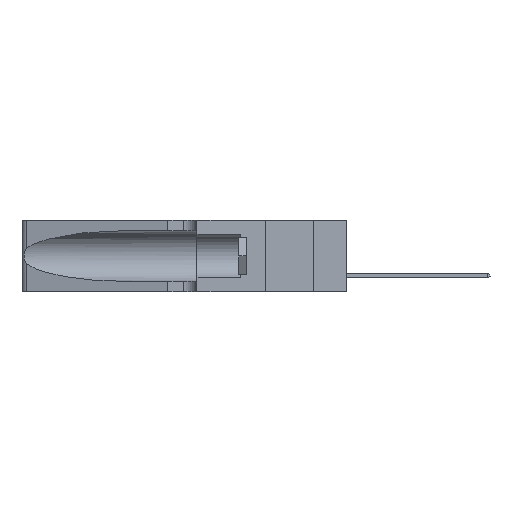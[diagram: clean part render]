
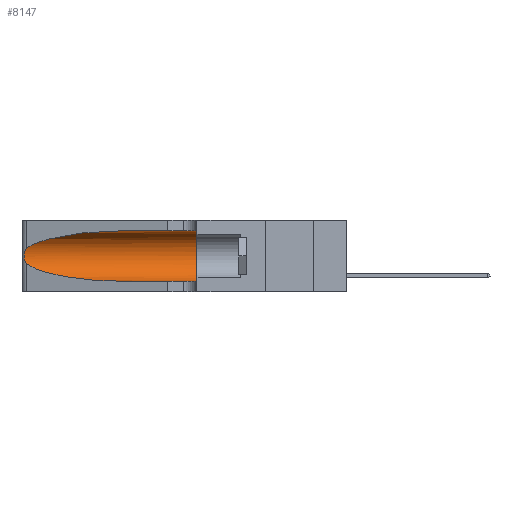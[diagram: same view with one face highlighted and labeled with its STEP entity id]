
A CAD part, left-side view. The second image highlights one B-rep face of the part: STEP entity #8147.
In plain terms, the highlighted cylindrical face has radius 3.308 mm (diameter 6.617 mm), a partial arc.
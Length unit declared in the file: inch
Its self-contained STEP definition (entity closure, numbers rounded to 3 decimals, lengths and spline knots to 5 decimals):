
#199 = FACE_OUTER_BOUND ( 'NONE', #6967, .T. ) ;
#1087 = CARTESIAN_POINT ( 'NONE',  ( 0.25487, 1.22718, 0.14631 ) ) ;
#1635 = CARTESIAN_POINT ( 'NONE',  ( 0.26018, 1.23835, 0.19895 ) ) ;
#2266 = ORIENTED_EDGE ( 'NONE', *, *, #4093, .T. ) ;
#2772 = CARTESIAN_POINT ( 'NONE',  ( 0.18966, 0.96281, 0.31525 ) ) ;
#2978 = CARTESIAN_POINT ( 'NONE',  ( 0.1305, 1.61858, 0.185 ) ) ;
#3443 = DIRECTION ( 'NONE',  ( 0., 1., 0. ) ) ;
#4093 = EDGE_CURVE ( 'NONE', #20057, #7512, #4691, .T. ) ;
#4691 = B_SPLINE_CURVE_WITH_KNOTS ( 'NONE', 3,
 ( #38558, #27583, #8957, #8781, #42356, #1635, #16392, #19839, #23615, #35313, #12773, #34964, #24465, #20704 ),
 .UNSPECIFIED., .F., .F.,
 ( 4, 2, 2, 2, 2, 2, 4 ),
 ( 0., 0.00027, 0.00053, 0.00107, 0.0016, 0.00187, 0.00214 ),
 .UNSPECIFIED. ) ;
#6109 = CARTESIAN_POINT ( 'NONE',  ( 0.25487, 1.22718, 0.22369 ) ) ;
#6454 = EDGE_CURVE ( 'NONE', #41723, #23977, #20462, .T. ) ;
#6967 = EDGE_LOOP ( 'NONE', ( #35686, #2266, #26978, #8843, #28911, #47625 ) ) ;
#7424 = CARTESIAN_POINT ( 'NONE',  ( 0.25487, 1.22718, 0.14631 ) ) ;
#7512 = VERTEX_POINT ( 'NONE', #7424 ) ;
#8147 = ADVANCED_FACE ( 'NONE', ( #199 ), #42537, .F. ) ;
#8781 = CARTESIAN_POINT ( 'NONE',  ( 0.25787, 1.23484, 0.2124 ) ) ;
#8843 = ORIENTED_EDGE ( 'NONE', *, *, #16078, .T. ) ;
#8957 = CARTESIAN_POINT ( 'NONE',  ( 0.25639, 1.23184, 0.21858 ) ) ;
#10916 = CARTESIAN_POINT ( 'NONE',  ( 0.1305, 0.35, 0.31525 ) ) ;
#12492 = DIRECTION ( 'NONE',  ( 0., -1., 0. ) ) ;
#12773 = CARTESIAN_POINT ( 'NONE',  ( 0.25789, 1.23486, 0.15765 ) ) ;
#12911 = LINE ( 'NONE', #35363, #38768 ) ;
#14139 = DIRECTION ( 'NONE',  ( 0., -1., 0. ) ) ;
#14301 = CARTESIAN_POINT ( 'NONE',  ( 0.1305, 0.35, 0.185 ) ) ;
#15576 = EDGE_CURVE ( 'NONE', #7512, #38236, #43875, .T. ) ;
#16078 = EDGE_CURVE ( 'NONE', #38236, #23977, #12911, .T. ) ;
#16392 = CARTESIAN_POINT ( 'NONE',  ( 0.26075, 1.23896, 0.19203 ) ) ;
#16457 = AXIS2_PLACEMENT_3D ( 'NONE', #14301, #3443, #17728 ) ;
#17728 = DIRECTION ( 'NONE',  ( 0., 0., 1. ) ) ;
#18174 = CARTESIAN_POINT ( 'NONE',  ( 0.2373, 1.15595, 0.28018 ) ) ;
#18338 = CARTESIAN_POINT ( 'NONE',  ( 0.1305, 0.72297, 0.05475 ) ) ;
#19839 = CARTESIAN_POINT ( 'NONE',  ( 0.26075, 1.23896, 0.178 ) ) ;
#19980 = AXIS2_PLACEMENT_3D ( 'NONE', #2978, #14139, #43865 ) ;
#20057 = VERTEX_POINT ( 'NONE', #6109 ) ;
#20462 = CIRCLE ( 'NONE', #16457, 0.13025 ) ;
#20704 = CARTESIAN_POINT ( 'NONE',  ( 0.25487, 1.22718, 0.14631 ) ) ;
#21912 = EDGE_CURVE ( 'NONE', #36188, #41723, #32035, .T. ) ;
#23615 = CARTESIAN_POINT ( 'NONE',  ( 0.26017, 1.23833, 0.17102 ) ) ;
#23977 = VERTEX_POINT ( 'NONE', #47162 ) ;
#24465 = CARTESIAN_POINT ( 'NONE',  ( 0.25555, 1.22993, 0.14849 ) ) ;
#25260 = CARTESIAN_POINT ( 'NONE',  ( 0.1305, 0.72297, 0.31525 ) ) ;
#26978 = ORIENTED_EDGE ( 'NONE', *, *, #15576, .T. ) ;
#27405 = EDGE_CURVE ( 'NONE', #36188, #20057, #35108, .T. ) ;
#27583 = CARTESIAN_POINT ( 'NONE',  ( 0.25555, 1.22994, 0.2215 ) ) ;
#28911 = ORIENTED_EDGE ( 'NONE', *, *, #6454, .F. ) ;
#31157 = DIRECTION ( 'NONE',  ( 0., -1., 0. ) ) ;
#32035 = LINE ( 'NONE', #41721, #46117 ) ;
#34964 = CARTESIAN_POINT ( 'NONE',  ( 0.25639, 1.23186, 0.15144 ) ) ;
#35108 =( BOUNDED_CURVE ( )  B_SPLINE_CURVE ( 3, ( #25260, #2772, #18174, #40537 ),
 .UNSPECIFIED., .F., .F. ) 
 B_SPLINE_CURVE_WITH_KNOTS ( ( 4, 4 ),
 ( 1.5708, 2.84003 ),
 .UNSPECIFIED. ) 
 CURVE ( )  GEOMETRIC_REPRESENTATION_ITEM ( )  RATIONAL_B_SPLINE_CURVE ( ( 1., 0.87, 0.87, 1. ) ) 
 REPRESENTATION_ITEM ( '' )  );
#35313 = CARTESIAN_POINT ( 'NONE',  ( 0.25856, 1.23593, 0.16098 ) ) ;
#35363 = CARTESIAN_POINT ( 'NONE',  ( 0.1305, 1.61858, 0.05475 ) ) ;
#35686 = ORIENTED_EDGE ( 'NONE', *, *, #27405, .T. ) ;
#36188 = VERTEX_POINT ( 'NONE', #47766 ) ;
#38236 = VERTEX_POINT ( 'NONE', #18338 ) ;
#38558 = CARTESIAN_POINT ( 'NONE',  ( 0.25487, 1.22718, 0.22369 ) ) ;
#38768 = VECTOR ( 'NONE', #12492, 39.37008 ) ;
#38838 = CARTESIAN_POINT ( 'NONE',  ( 0.2373, 1.15595, 0.08982 ) ) ;
#40537 = CARTESIAN_POINT ( 'NONE',  ( 0.25487, 1.22718, 0.22369 ) ) ;
#41721 = CARTESIAN_POINT ( 'NONE',  ( 0.1305, 1.61858, 0.31525 ) ) ;
#41723 = VERTEX_POINT ( 'NONE', #10916 ) ;
#42013 = CARTESIAN_POINT ( 'NONE',  ( 0.1305, 0.72297, 0.05475 ) ) ;
#42356 = CARTESIAN_POINT ( 'NONE',  ( 0.25854, 1.2359, 0.20912 ) ) ;
#42481 = CARTESIAN_POINT ( 'NONE',  ( 0.18966, 0.96281, 0.05475 ) ) ;
#42537 = CYLINDRICAL_SURFACE ( 'NONE', #19980, 0.13025 ) ;
#43865 = DIRECTION ( 'NONE',  ( 0., 0., -1. ) ) ;
#43875 =( BOUNDED_CURVE ( )  B_SPLINE_CURVE ( 3, ( #1087, #38838, #42481, #42013 ),
 .UNSPECIFIED., .F., .F. ) 
 B_SPLINE_CURVE_WITH_KNOTS ( ( 4, 4 ),
 ( 3.44316, 4.71239 ),
 .UNSPECIFIED. ) 
 CURVE ( )  GEOMETRIC_REPRESENTATION_ITEM ( )  RATIONAL_B_SPLINE_CURVE ( ( 1., 0.87, 0.87, 1. ) ) 
 REPRESENTATION_ITEM ( '' )  );
#46117 = VECTOR ( 'NONE', #31157, 39.37008 ) ;
#47162 = CARTESIAN_POINT ( 'NONE',  ( 0.1305, 0.35, 0.05475 ) ) ;
#47625 = ORIENTED_EDGE ( 'NONE', *, *, #21912, .F. ) ;
#47766 = CARTESIAN_POINT ( 'NONE',  ( 0.1305, 0.72297, 0.31525 ) ) ;
